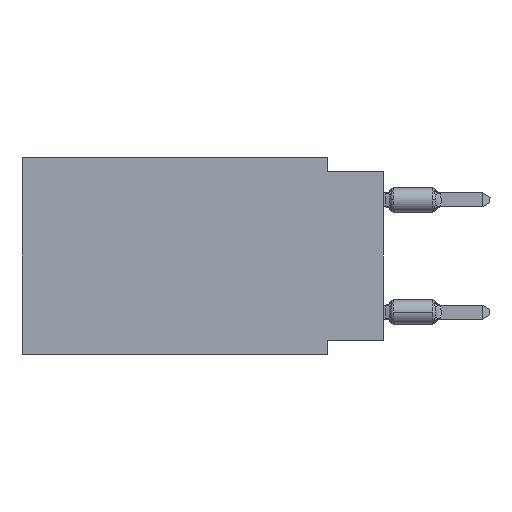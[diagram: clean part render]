
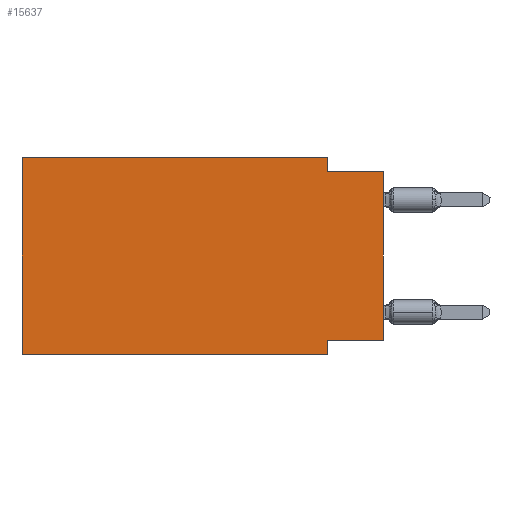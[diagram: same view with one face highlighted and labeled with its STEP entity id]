
A CAD part, left-side view. The second image highlights one B-rep face of the part: STEP entity #15637.
In plain terms, the highlighted planar face has unit normal (-1, 0, 0).
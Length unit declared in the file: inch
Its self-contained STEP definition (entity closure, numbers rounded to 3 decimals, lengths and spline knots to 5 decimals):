
#112 = CARTESIAN_POINT ( 'NONE',  ( 0., 0.645, -0.35 ) ) ;
#1014 = VERTEX_POINT ( 'NONE', #33237 ) ;
#2430 = CARTESIAN_POINT ( 'NONE',  ( 0., 0.1, -0.35 ) ) ;
#2613 = DIRECTION ( 'NONE',  ( 0., -1., 0. ) ) ;
#3115 = VECTOR ( 'NONE', #32174, 39.37008 ) ;
#3828 = DIRECTION ( 'NONE',  ( 0., 0., 1. ) ) ;
#4961 = CARTESIAN_POINT ( 'NONE',  ( 0., 0., -0.025 ) ) ;
#5551 = DIRECTION ( 'NONE',  ( 0., -1., 0. ) ) ;
#5916 = CARTESIAN_POINT ( 'NONE',  ( 0., 0.645, 0. ) ) ;
#6398 = CARTESIAN_POINT ( 'NONE',  ( 0., 0., 0. ) ) ;
#6887 = DIRECTION ( 'NONE',  ( 0., 1., 0. ) ) ;
#7568 = LINE ( 'NONE', #33957, #3115 ) ;
#7584 = VECTOR ( 'NONE', #3828, 39.37008 ) ;
#7748 = LINE ( 'NONE', #4961, #9521 ) ;
#8025 = CARTESIAN_POINT ( 'NONE',  ( 0., 0.1, 0. ) ) ;
#8698 = LINE ( 'NONE', #5916, #14533 ) ;
#8954 = VERTEX_POINT ( 'NONE', #35180 ) ;
#8992 = EDGE_CURVE ( 'NONE', #22378, #33235, #36507, .T. ) ;
#9188 = CARTESIAN_POINT ( 'NONE',  ( 0., 0., -0.325 ) ) ;
#9205 = EDGE_CURVE ( 'NONE', #20373, #1014, #8698, .T. ) ;
#9521 = VECTOR ( 'NONE', #2613, 39.37008 ) ;
#9933 = VECTOR ( 'NONE', #6887, 39.37008 ) ;
#10921 = DIRECTION ( 'NONE',  ( 0., 0., -1. ) ) ;
#11427 = ORIENTED_EDGE ( 'NONE', *, *, #8992, .T. ) ;
#12160 = EDGE_CURVE ( 'NONE', #22378, #18645, #33867, .T. ) ;
#12225 = ORIENTED_EDGE ( 'NONE', *, *, #37547, .T. ) ;
#12675 = VERTEX_POINT ( 'NONE', #19217 ) ;
#13256 = ORIENTED_EDGE ( 'NONE', *, *, #33189, .F. ) ;
#13996 = CARTESIAN_POINT ( 'NONE',  ( 0., 0.645, 0. ) ) ;
#14491 = VECTOR ( 'NONE', #10921, 39.37008 ) ;
#14533 = VECTOR ( 'NONE', #35845, 39.37008 ) ;
#15637 = ADVANCED_FACE ( 'NONE', ( #26573 ), #26376, .F. ) ;
#17837 = ORIENTED_EDGE ( 'NONE', *, *, #19414, .F. ) ;
#18645 = VERTEX_POINT ( 'NONE', #24464 ) ;
#19217 = CARTESIAN_POINT ( 'NONE',  ( 0., 0.1, -0.025 ) ) ;
#19414 = EDGE_CURVE ( 'NONE', #1014, #8954, #7568, .T. ) ;
#19422 = EDGE_CURVE ( 'NONE', #18645, #37172, #37865, .T. ) ;
#20273 = DIRECTION ( 'NONE',  ( 0., 0., -1. ) ) ;
#20373 = VERTEX_POINT ( 'NONE', #112 ) ;
#20960 = LINE ( 'NONE', #26447, #37849 ) ;
#21631 = ORIENTED_EDGE ( 'NONE', *, *, #12160, .F. ) ;
#22378 = VERTEX_POINT ( 'NONE', #9188 ) ;
#24157 = AXIS2_PLACEMENT_3D ( 'NONE', #13996, #38560, #31893 ) ;
#24464 = CARTESIAN_POINT ( 'NONE',  ( 0., 0.1, -0.325 ) ) ;
#26376 = PLANE ( 'NONE',  #24157 ) ;
#26447 = CARTESIAN_POINT ( 'NONE',  ( 0., 0.645, -0.35 ) ) ;
#26573 = FACE_OUTER_BOUND ( 'NONE', #34341, .T. ) ;
#26954 = ORIENTED_EDGE ( 'NONE', *, *, #9205, .F. ) ;
#27126 = ORIENTED_EDGE ( 'NONE', *, *, #36715, .F. ) ;
#29857 = CARTESIAN_POINT ( 'NONE',  ( 0., 0.1, -0.35 ) ) ;
#31893 = DIRECTION ( 'NONE',  ( 0., 0., -1. ) ) ;
#32174 = DIRECTION ( 'NONE',  ( 0., -1., 0. ) ) ;
#33189 = EDGE_CURVE ( 'NONE', #8954, #12675, #35372, .T. ) ;
#33235 = VERTEX_POINT ( 'NONE', #37740 ) ;
#33237 = CARTESIAN_POINT ( 'NONE',  ( 0., 0.645, 0. ) ) ;
#33675 = CARTESIAN_POINT ( 'NONE',  ( 0., 0., -0.325 ) ) ;
#33867 = LINE ( 'NONE', #33675, #9933 ) ;
#33946 = VECTOR ( 'NONE', #20273, 39.37008 ) ;
#33957 = CARTESIAN_POINT ( 'NONE',  ( 0., 0.645, 0. ) ) ;
#34341 = EDGE_LOOP ( 'NONE', ( #11427, #27126, #13256, #17837, #26954, #12225, #35172, #21631 ) ) ;
#35172 = ORIENTED_EDGE ( 'NONE', *, *, #19422, .F. ) ;
#35180 = CARTESIAN_POINT ( 'NONE',  ( 0., 0.1, 0. ) ) ;
#35372 = LINE ( 'NONE', #8025, #33946 ) ;
#35845 = DIRECTION ( 'NONE',  ( 0., 0., 1. ) ) ;
#36507 = LINE ( 'NONE', #6398, #7584 ) ;
#36715 = EDGE_CURVE ( 'NONE', #12675, #33235, #7748, .T. ) ;
#37172 = VERTEX_POINT ( 'NONE', #29857 ) ;
#37547 = EDGE_CURVE ( 'NONE', #20373, #37172, #20960, .T. ) ;
#37740 = CARTESIAN_POINT ( 'NONE',  ( 0., 0., -0.025 ) ) ;
#37849 = VECTOR ( 'NONE', #5551, 39.37008 ) ;
#37865 = LINE ( 'NONE', #2430, #14491 ) ;
#38560 = DIRECTION ( 'NONE',  ( 1., 0., 0. ) ) ;
